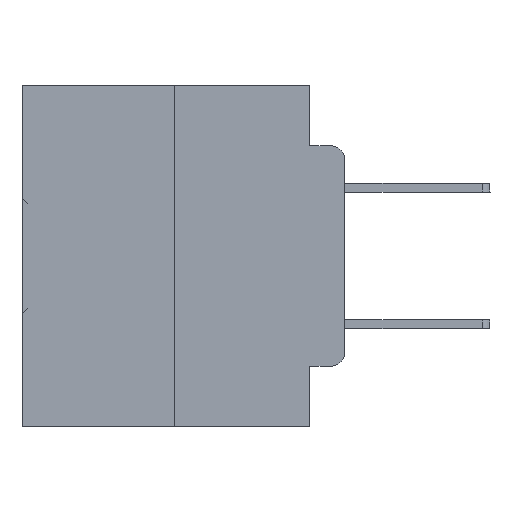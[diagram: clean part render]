
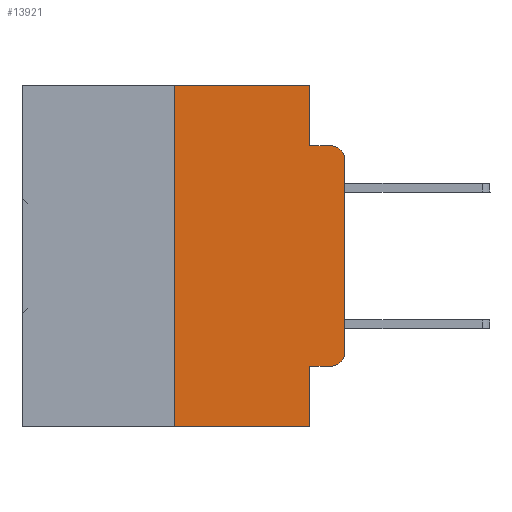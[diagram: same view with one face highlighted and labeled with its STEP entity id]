
A CAD part, left-side view. The second image highlights one B-rep face of the part: STEP entity #13921.
In plain terms, the highlighted planar face has unit normal (-1, 0, 0).
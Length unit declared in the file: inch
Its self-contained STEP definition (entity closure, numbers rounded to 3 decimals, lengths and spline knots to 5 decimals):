
#444 = ORIENTED_EDGE ( 'NONE', *, *, #25210, .F. ) ;
#589 = DIRECTION ( 'NONE',  ( -1., 0., 0. ) ) ;
#614 = ORIENTED_EDGE ( 'NONE', *, *, #4295, .T. ) ;
#1294 = VERTEX_POINT ( 'NONE', #15732 ) ;
#1716 = CARTESIAN_POINT ( 'NONE',  ( 0., 0.25, 0. ) ) ;
#1903 = AXIS2_PLACEMENT_3D ( 'NONE', #14190, #34228, #8567 ) ;
#3233 = EDGE_CURVE ( 'NONE', #12403, #19718, #10283, .T. ) ;
#4110 = LINE ( 'NONE', #12716, #17277 ) ;
#4295 = EDGE_CURVE ( 'NONE', #4649, #1294, #28076, .T. ) ;
#4649 = VERTEX_POINT ( 'NONE', #7482 ) ;
#5015 = LINE ( 'NONE', #16057, #32278 ) ;
#5116 = ORIENTED_EDGE ( 'NONE', *, *, #3233, .F. ) ;
#5532 = ORIENTED_EDGE ( 'NONE', *, *, #14365, .T. ) ;
#5625 = EDGE_CURVE ( 'NONE', #26154, #19718, #34016, .T. ) ;
#5856 = LINE ( 'NONE', #8842, #30886 ) ;
#6276 = CARTESIAN_POINT ( 'NONE',  ( 0., 0.25, -0.5 ) ) ;
#6578 = CARTESIAN_POINT ( 'NONE',  ( 0., 0.473, 0. ) ) ;
#6761 = ORIENTED_EDGE ( 'NONE', *, *, #5625, .T. ) ;
#7442 = DIRECTION ( 'NONE',  ( 0., -1., 0. ) ) ;
#7482 = CARTESIAN_POINT ( 'NONE',  ( 0., 0., -0.1085 ) ) ;
#7528 = LINE ( 'NONE', #13330, #31983 ) ;
#8140 = AXIS2_PLACEMENT_3D ( 'NONE', #9063, #8694, #20297 ) ;
#8359 = CARTESIAN_POINT ( 'NONE',  ( 0., 0.473, -0.5 ) ) ;
#8567 = DIRECTION ( 'NONE',  ( 0., 0., -1. ) ) ;
#8694 = DIRECTION ( 'NONE',  ( 1., 0., 0. ) ) ;
#8842 = CARTESIAN_POINT ( 'NONE',  ( 0., 0.051, -0.4115 ) ) ;
#9063 = CARTESIAN_POINT ( 'NONE',  ( 0., 0.473, 0. ) ) ;
#10283 = LINE ( 'NONE', #32962, #12298 ) ;
#12096 = VERTEX_POINT ( 'NONE', #19233 ) ;
#12298 = VECTOR ( 'NONE', #33713, 39.37008 ) ;
#12403 = VERTEX_POINT ( 'NONE', #31573 ) ;
#12648 = CARTESIAN_POINT ( 'NONE',  ( 0., 0.051, -0.5 ) ) ;
#12716 = CARTESIAN_POINT ( 'NONE',  ( 0., 0.051, 0. ) ) ;
#13042 = EDGE_CURVE ( 'NONE', #34180, #4649, #7528, .T. ) ;
#13330 = CARTESIAN_POINT ( 'NONE',  ( 0., 0., 0. ) ) ;
#13906 = ORIENTED_EDGE ( 'NONE', *, *, #21422, .T. ) ;
#13921 = ADVANCED_FACE ( 'NONE', ( #14316 ), #20676, .F. ) ;
#14190 = CARTESIAN_POINT ( 'NONE',  ( 0., 0.02, -0.3915 ) ) ;
#14316 = FACE_OUTER_BOUND ( 'NONE', #29787, .T. ) ;
#14365 = EDGE_CURVE ( 'NONE', #12403, #12096, #5856, .T. ) ;
#14536 = CARTESIAN_POINT ( 'NONE',  ( 0., 0.25, 0. ) ) ;
#14639 = DIRECTION ( 'NONE',  ( 0., -1., 0. ) ) ;
#14706 = CARTESIAN_POINT ( 'NONE',  ( 0., 0.051, 0. ) ) ;
#15058 = CARTESIAN_POINT ( 'NONE',  ( 0., 0.051, -0.0885 ) ) ;
#15210 = VERTEX_POINT ( 'NONE', #15058 ) ;
#15732 = CARTESIAN_POINT ( 'NONE',  ( 0., 0.02, -0.0885 ) ) ;
#16057 = CARTESIAN_POINT ( 'NONE',  ( 0., 0.051, -0.0885 ) ) ;
#17255 = ORIENTED_EDGE ( 'NONE', *, *, #19416, .F. ) ;
#17277 = VECTOR ( 'NONE', #24140, 39.37008 ) ;
#17577 = CARTESIAN_POINT ( 'NONE',  ( 0., 0., -0.3915 ) ) ;
#18019 = CIRCLE ( 'NONE', #1903, 0.02 ) ;
#18057 = EDGE_CURVE ( 'NONE', #15210, #1294, #5015, .T. ) ;
#18730 = DIRECTION ( 'NONE',  ( 0., 0., 1. ) ) ;
#19233 = CARTESIAN_POINT ( 'NONE',  ( 0., 0.02, -0.4115 ) ) ;
#19416 = EDGE_CURVE ( 'NONE', #26154, #27402, #33558, .T. ) ;
#19718 = VERTEX_POINT ( 'NONE', #12648 ) ;
#19776 = DIRECTION ( 'NONE',  ( 0., -1., 0. ) ) ;
#20297 = DIRECTION ( 'NONE',  ( 0., 0., -1. ) ) ;
#20620 = LINE ( 'NONE', #6578, #36547 ) ;
#20676 = PLANE ( 'NONE',  #8140 ) ;
#20805 = DIRECTION ( 'NONE',  ( 0., -1., 0. ) ) ;
#21422 = EDGE_CURVE ( 'NONE', #12096, #34180, #18019, .T. ) ;
#23019 = VECTOR ( 'NONE', #19776, 39.37008 ) ;
#24140 = DIRECTION ( 'NONE',  ( 0., 0., -1. ) ) ;
#25094 = VECTOR ( 'NONE', #18730, 39.37008 ) ;
#25210 = EDGE_CURVE ( 'NONE', #25944, #15210, #4110, .T. ) ;
#25944 = VERTEX_POINT ( 'NONE', #14706 ) ;
#26154 = VERTEX_POINT ( 'NONE', #6276 ) ;
#26161 = ORIENTED_EDGE ( 'NONE', *, *, #28490, .F. ) ;
#27402 = VERTEX_POINT ( 'NONE', #14536 ) ;
#28076 = CIRCLE ( 'NONE', #33476, 0.02 ) ;
#28490 = EDGE_CURVE ( 'NONE', #27402, #25944, #20620, .T. ) ;
#28675 = DIRECTION ( 'NONE',  ( 0., 0., -1. ) ) ;
#29787 = EDGE_LOOP ( 'NONE', ( #36808, #614, #30982, #444, #26161, #17255, #6761, #5116, #5532, #13906 ) ) ;
#30886 = VECTOR ( 'NONE', #14639, 39.37008 ) ;
#30982 = ORIENTED_EDGE ( 'NONE', *, *, #18057, .F. ) ;
#31573 = CARTESIAN_POINT ( 'NONE',  ( 0., 0.051, -0.4115 ) ) ;
#31983 = VECTOR ( 'NONE', #33197, 39.37008 ) ;
#32278 = VECTOR ( 'NONE', #7442, 39.37008 ) ;
#32962 = CARTESIAN_POINT ( 'NONE',  ( 0., 0.051, 0. ) ) ;
#33197 = DIRECTION ( 'NONE',  ( 0., 0., 1. ) ) ;
#33476 = AXIS2_PLACEMENT_3D ( 'NONE', #34481, #589, #28675 ) ;
#33558 = LINE ( 'NONE', #1716, #25094 ) ;
#33713 = DIRECTION ( 'NONE',  ( 0., 0., -1. ) ) ;
#34016 = LINE ( 'NONE', #8359, #23019 ) ;
#34180 = VERTEX_POINT ( 'NONE', #17577 ) ;
#34228 = DIRECTION ( 'NONE',  ( -1., 0., 0. ) ) ;
#34481 = CARTESIAN_POINT ( 'NONE',  ( 0., 0.02, -0.1085 ) ) ;
#36547 = VECTOR ( 'NONE', #20805, 39.37008 ) ;
#36808 = ORIENTED_EDGE ( 'NONE', *, *, #13042, .T. ) ;
